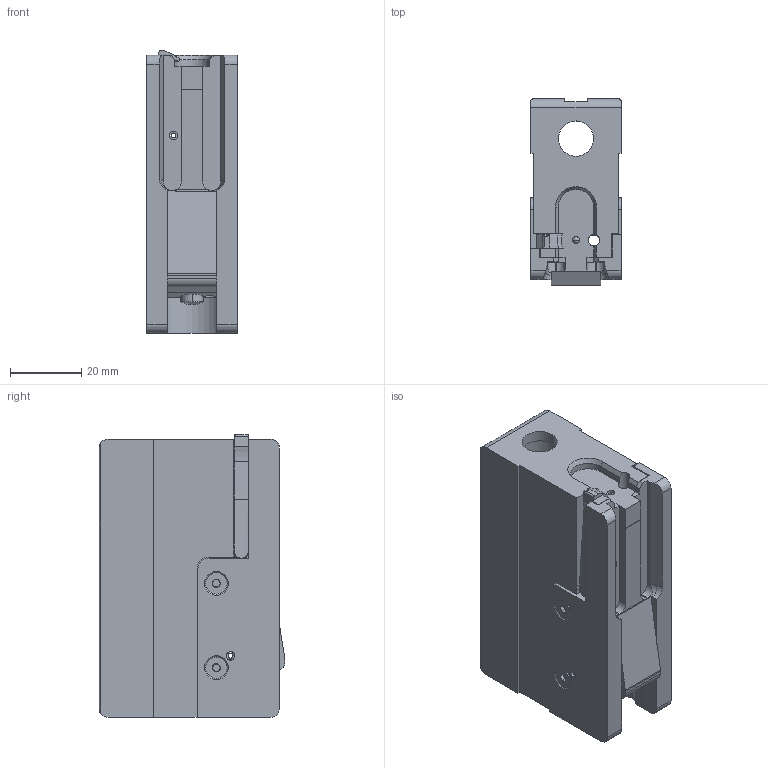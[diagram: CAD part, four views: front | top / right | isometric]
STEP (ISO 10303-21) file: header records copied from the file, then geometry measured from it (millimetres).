
FILE_DESCRIPTION (( 'STEP AP214' ), '1' );
FILE_NAME ('PPDW9 V3 Bolt split 2 piece.STEP', '2020-12-28T03:16:01', ( '' ), ( '' ), 'SwSTEP 2.0', 'SolidWorks 2020', '' );
FILE_SCHEMA (( 'AUTOMOTIVE_DESIGN' ));
Length unit declared in the file: inch
Products named in the file (9): Extractor spring 9657K256_9657K256; M3 x 6mm FHSHS 91294A126_BLACK_91294A126; P38 Firing Pin; Beretta 92 scanned extractor; 3-32 92383A859_TYPE 420 STAINLESS STEEL SLOTTED SPRING PIN_92383A859; PPDW9 V3 Bolt split upper; PPDW9 V3 Bolt split bottom; PPDW9 V3 Bolt split 2 piece; Firing Pin Spring 9657K242_9657K242
Assembly tree (12 placements, depth 2):
  PPDW9 V3 Bolt split 2 piece
    PPDW9 V3 Bolt split bottom
    PPDW9 V3 Bolt split upper
    M3 x 6mm FHSHS 91294A126_BLACK_91294A126  x4
    3-32 92383A859_TYPE 420 STAINLESS STEEL SLOTTED SPRING PIN_92383A859  x2
    Beretta 92 scanned extractor
    P38 Firing Pin
    Firing Pin Spring 9657K242_9657K242
    Extractor spring 9657K256_9657K256
Bounding box: 25.4 x 52.32 x 79.57 mm (x, y, z)
Volume: 77342.2 mm3; surface area: 31610.9 mm2
Topology: 12 solids, 12 shells, 593 faces, 1576 edges, 1000 vertices
Faces by surface type: cylinder 264, plane 196, cone 77, bspline 42, torus 8, sphere 6
Entity records: 22879 total; most frequent: CARTESIAN_POINT 12553, ORIENTED_EDGE 2150, DIRECTION 1919, EDGE_CURVE 1075, VERTEX_POINT 690, AXIS2_PLACEMENT_3D 678, LINE 563, VECTOR 563
